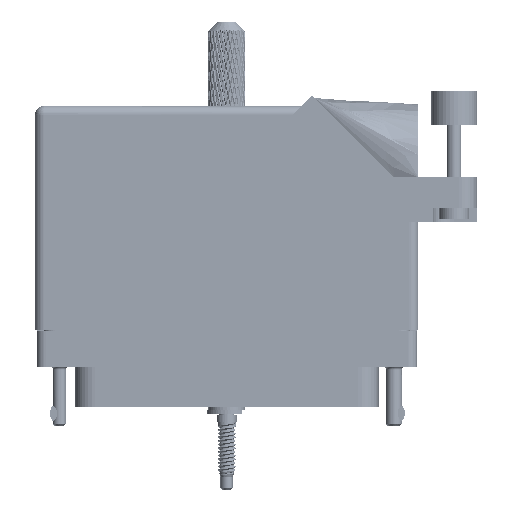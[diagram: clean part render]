
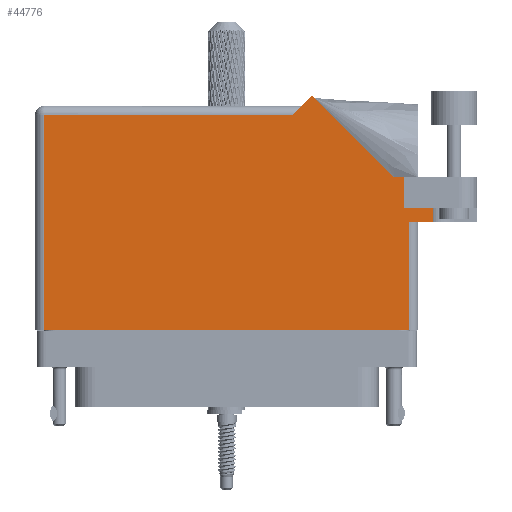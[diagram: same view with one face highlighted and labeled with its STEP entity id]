
A CAD part, front view. The second image highlights one B-rep face of the part: STEP entity #44776.
In plain terms, the highlighted face is planar.
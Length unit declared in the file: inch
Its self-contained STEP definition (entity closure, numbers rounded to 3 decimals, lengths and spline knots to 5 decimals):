
#353 = VECTOR ( 'NONE', #37978, 39.37008 ) ;
#1354 = VECTOR ( 'NONE', #123709, 39.37008 ) ;
#1949 = VERTEX_POINT ( 'NONE', #103942 ) ;
#3677 = VERTEX_POINT ( 'NONE', #15899 ) ;
#10057 = ORIENTED_EDGE ( 'NONE', *, *, #78400, .T. ) ;
#10258 = CARTESIAN_POINT ( 'NONE',  ( 1.4075, 0.731, 0.455 ) ) ;
#10676 = LINE ( 'NONE', #60857, #99076 ) ;
#11150 = VERTEX_POINT ( 'NONE', #80599 ) ;
#11346 = EDGE_CURVE ( 'NONE', #3677, #11150, #55138, .T. ) ;
#12239 = CARTESIAN_POINT ( 'NONE',  ( 0.451, 1.368, 0.455 ) ) ;
#12487 = ORIENTED_EDGE ( 'NONE', *, *, #104301, .T. ) ;
#13366 = EDGE_CURVE ( 'NONE', #113911, #108921, #10676, .T. ) ;
#15071 = DIRECTION ( 'NONE',  ( 1., 0., 0. ) ) ;
#15899 = CARTESIAN_POINT ( 'NONE',  ( 1.206, 0.731, 0.455 ) ) ;
#17127 = VERTEX_POINT ( 'NONE', #79136 ) ;
#18084 = ORIENTED_EDGE ( 'NONE', *, *, #67743, .T. ) ;
#25793 = VECTOR ( 'NONE', #91910, 39.37008 ) ;
#34769 = CARTESIAN_POINT ( 'NONE',  ( 1.14042, 0.944, 0.455 ) ) ;
#36256 = DIRECTION ( 'NONE',  ( 1., 0., 0. ) ) ;
#37640 = CARTESIAN_POINT ( 'NONE',  ( 0.513, 1.43, 0.455 ) ) ;
#37978 = DIRECTION ( 'NONE',  ( -1., 0., 0. ) ) ;
#38536 = EDGE_CURVE ( 'NONE', #123741, #74832, #50624, .T. ) ;
#40953 = CARTESIAN_POINT ( 'NONE',  ( -1.306, 1.368, 0.455 ) ) ;
#41455 = CARTESIAN_POINT ( 'NONE',  ( 1.4075, 0.637, 0.455 ) ) ;
#41955 = VECTOR ( 'NONE', #94374, 39.37008 ) ;
#42256 = ORIENTED_EDGE ( 'NONE', *, *, #76869, .T. ) ;
#42550 = EDGE_CURVE ( 'NONE', #104175, #123741, #114909, .T. ) ;
#42987 = VERTEX_POINT ( 'NONE', #119185 ) ;
#44776 = ADVANCED_FACE ( 'NONE', ( #55777 ), #85985, .F. ) ;
#46743 = VECTOR ( 'NONE', #36256, 39.37008 ) ;
#50624 = LINE ( 'NONE', #40953, #116915 ) ;
#54660 = EDGE_CURVE ( 'NONE', #1949, #42987, #123168, .T. ) ;
#55138 = LINE ( 'NONE', #124600, #41955 ) ;
#55777 = FACE_OUTER_BOUND ( 'NONE', #85222, .T. ) ;
#60857 = CARTESIAN_POINT ( 'NONE',  ( 1.4075, 1.06177, 0.455 ) ) ;
#61191 = EDGE_CURVE ( 'NONE', #42987, #91083, #100323, .T. ) ;
#64147 = DIRECTION ( 'NONE',  ( 0., 0., -1. ) ) ;
#66043 = CARTESIAN_POINT ( 'NONE',  ( -1.306, 1.43, 0.455 ) ) ;
#67743 = EDGE_CURVE ( 'NONE', #11150, #17127, #68271, .T. ) ;
#68271 = LINE ( 'NONE', #125552, #353 ) ;
#73203 = VECTOR ( 'NONE', #74050, 39.37008 ) ;
#74050 = DIRECTION ( 'NONE',  ( -0.707, 0.707, 0. ) ) ;
#74832 = VERTEX_POINT ( 'NONE', #77455 ) ;
#76869 = EDGE_CURVE ( 'NONE', #17127, #104175, #122945, .T. ) ;
#77455 = CARTESIAN_POINT ( 'NONE',  ( -1.244, 1.368, 0.455 ) ) ;
#78400 = EDGE_CURVE ( 'NONE', #74832, #1949, #95377, .T. ) ;
#79136 = CARTESIAN_POINT ( 'NONE',  ( 1.14042, 0.944, 0.455 ) ) ;
#79525 = DIRECTION ( 'NONE',  ( 0., -1., 0. ) ) ;
#80599 = CARTESIAN_POINT ( 'NONE',  ( 1.206, 0.944, 0.455 ) ) ;
#85222 = EDGE_LOOP ( 'NONE', ( #117347, #123511, #12487, #97281, #125240, #118134, #18084, #42256, #95662, #120186, #10057 ) ) ;
#85707 = CARTESIAN_POINT ( 'NONE',  ( -1.244, -0.1, 0.455 ) ) ;
#85985 = PLANE ( 'NONE',  #112154 ) ;
#91083 = VERTEX_POINT ( 'NONE', #109068 ) ;
#91137 = DIRECTION ( 'NONE',  ( -1., 0., 0. ) ) ;
#91910 = DIRECTION ( 'NONE',  ( 1., 0., 0. ) ) ;
#92292 = CARTESIAN_POINT ( 'NONE',  ( -1.306, -0.1, 0.455 ) ) ;
#94213 = CARTESIAN_POINT ( 'NONE',  ( 1.306, 0.637, 0.455 ) ) ;
#94374 = DIRECTION ( 'NONE',  ( 0., 1., 0. ) ) ;
#95377 = LINE ( 'NONE', #85707, #1354 ) ;
#95640 = DIRECTION ( 'NONE',  ( -1., 0., 0. ) ) ;
#95662 = ORIENTED_EDGE ( 'NONE', *, *, #42550, .T. ) ;
#95786 = CARTESIAN_POINT ( 'NONE',  ( 0.58371, 1.50071, 0.455 ) ) ;
#96633 = EDGE_CURVE ( 'NONE', #3677, #113911, #101572, .T. ) ;
#97281 = ORIENTED_EDGE ( 'NONE', *, *, #13366, .F. ) ;
#99076 = VECTOR ( 'NONE', #79525, 39.37008 ) ;
#100323 = LINE ( 'NONE', #110620, #121581 ) ;
#101572 = LINE ( 'NONE', #111860, #25793 ) ;
#103942 = CARTESIAN_POINT ( 'NONE',  ( -1.244, -0.1, 0.455 ) ) ;
#104175 = VERTEX_POINT ( 'NONE', #95786 ) ;
#104301 = EDGE_CURVE ( 'NONE', #91083, #108921, #124438, .T. ) ;
#106513 = DIRECTION ( 'NONE',  ( -0.707, -0.707, 0. ) ) ;
#108921 = VERTEX_POINT ( 'NONE', #41455 ) ;
#109016 = VECTOR ( 'NONE', #15071, 39.37008 ) ;
#109068 = CARTESIAN_POINT ( 'NONE',  ( 1.244, 0.637, 0.455 ) ) ;
#109339 = DIRECTION ( 'NONE',  ( 0., 1., 0. ) ) ;
#110132 = VECTOR ( 'NONE', #106513, 39.37008 ) ;
#110620 = CARTESIAN_POINT ( 'NONE',  ( 1.244, 0.637, 0.455 ) ) ;
#111860 = CARTESIAN_POINT ( 'NONE',  ( 1.206, 0.731, 0.455 ) ) ;
#112154 = AXIS2_PLACEMENT_3D ( 'NONE', #66043, #64147, #95640 ) ;
#113911 = VERTEX_POINT ( 'NONE', #10258 ) ;
#114909 = LINE ( 'NONE', #37640, #110132 ) ;
#116915 = VECTOR ( 'NONE', #91137, 39.37008 ) ;
#117347 = ORIENTED_EDGE ( 'NONE', *, *, #54660, .T. ) ;
#118134 = ORIENTED_EDGE ( 'NONE', *, *, #11346, .T. ) ;
#119185 = CARTESIAN_POINT ( 'NONE',  ( 1.244, -0.1, 0.455 ) ) ;
#120186 = ORIENTED_EDGE ( 'NONE', *, *, #38536, .T. ) ;
#121581 = VECTOR ( 'NONE', #109339, 39.37008 ) ;
#122945 = LINE ( 'NONE', #34769, #73203 ) ;
#123168 = LINE ( 'NONE', #92292, #109016 ) ;
#123511 = ORIENTED_EDGE ( 'NONE', *, *, #61191, .T. ) ;
#123709 = DIRECTION ( 'NONE',  ( 0., -1., 0. ) ) ;
#123741 = VERTEX_POINT ( 'NONE', #12239 ) ;
#124438 = LINE ( 'NONE', #94213, #46743 ) ;
#124600 = CARTESIAN_POINT ( 'NONE',  ( 1.206, 0.731, 0.455 ) ) ;
#125240 = ORIENTED_EDGE ( 'NONE', *, *, #96633, .F. ) ;
#125552 = CARTESIAN_POINT ( 'NONE',  ( 1.706, 0.944, 0.455 ) ) ;
